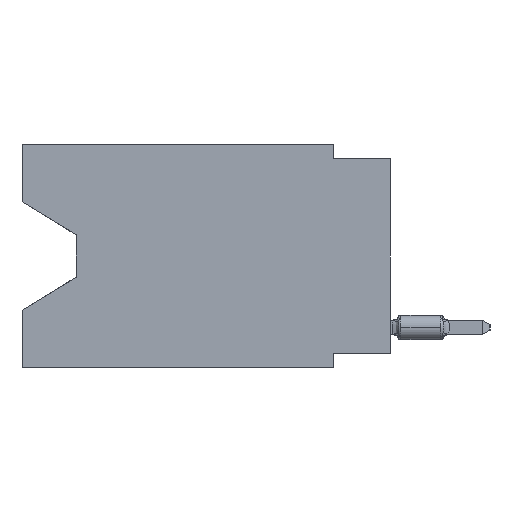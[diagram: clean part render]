
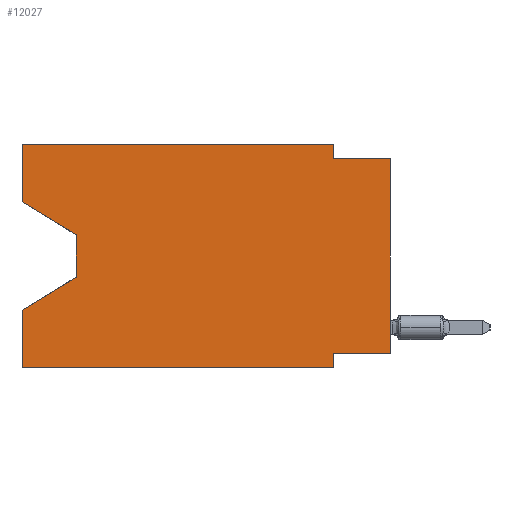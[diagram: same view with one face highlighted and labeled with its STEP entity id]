
A CAD part, left-side view. The second image highlights one B-rep face of the part: STEP entity #12027.
In plain terms, the highlighted planar face has unit normal (-1, 0, 0).
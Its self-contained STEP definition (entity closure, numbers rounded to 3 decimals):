
#24 = EDGE_CURVE ( 'NONE', #1278, #14343, #8043, .T. ) ;
#43 = CARTESIAN_POINT ( 'NONE',  ( 0., 13.97, -4.013 ) ) ;
#443 = ORIENTED_EDGE ( 'NONE', *, *, #35707, .T. ) ;
#449 = CARTESIAN_POINT ( 'NONE',  ( 0., 16.383, 0. ) ) ;
#1278 = VERTEX_POINT ( 'NONE', #25977 ) ;
#2198 = EDGE_CURVE ( 'NONE', #7456, #37600, #7278, .T. ) ;
#2207 = CARTESIAN_POINT ( 'NONE',  ( 0., 0., -0.635 ) ) ;
#2524 = EDGE_CURVE ( 'NONE', #11886, #22680, #27853, .T. ) ;
#3757 = LINE ( 'NONE', #13582, #19333 ) ;
#3829 = CARTESIAN_POINT ( 'NONE',  ( 0., 16.383, 0. ) ) ;
#4867 = LINE ( 'NONE', #16877, #7939 ) ;
#5204 = EDGE_CURVE ( 'NONE', #37988, #37600, #23819, .T. ) ;
#5759 = VECTOR ( 'NONE', #25154, 1000. ) ;
#5802 = ORIENTED_EDGE ( 'NONE', *, *, #24, .F. ) ;
#7278 = LINE ( 'NONE', #22023, #5759 ) ;
#7456 = VERTEX_POINT ( 'NONE', #24788 ) ;
#7939 = VECTOR ( 'NONE', #10017, 1000. ) ;
#8043 = LINE ( 'NONE', #32368, #18866 ) ;
#8679 = VERTEX_POINT ( 'NONE', #33979 ) ;
#8812 = LINE ( 'NONE', #21389, #20976 ) ;
#9081 = LINE ( 'NONE', #29108, #38575 ) ;
#9101 = LINE ( 'NONE', #24217, #18925 ) ;
#9214 = DIRECTION ( 'NONE',  ( 0., 0., -1. ) ) ;
#10017 = DIRECTION ( 'NONE',  ( 0., -0.855, -0.519 ) ) ;
#11312 = EDGE_CURVE ( 'NONE', #11886, #8679, #4867, .T. ) ;
#11886 = VERTEX_POINT ( 'NONE', #22898 ) ;
#12027 = ADVANCED_FACE ( 'NONE', ( #29937 ), #12666, .F. ) ;
#12666 = PLANE ( 'NONE',  #12703 ) ;
#12680 = CARTESIAN_POINT ( 'NONE',  ( 0., 2.54, -9.271 ) ) ;
#12703 = AXIS2_PLACEMENT_3D ( 'NONE', #449, #24246, #30527 ) ;
#13582 = CARTESIAN_POINT ( 'NONE',  ( 0., 0., -9.271 ) ) ;
#14343 = VERTEX_POINT ( 'NONE', #19339 ) ;
#14883 = VECTOR ( 'NONE', #36579, 1000. ) ;
#15309 = DIRECTION ( 'NONE',  ( 0., 0., 1. ) ) ;
#15353 = EDGE_LOOP ( 'NONE', ( #17076, #443, #38571, #5802, #32277, #36869, #23193, #25062, #33056, #28447, #30526, #15473 ) ) ;
#15473 = ORIENTED_EDGE ( 'NONE', *, *, #2524, .F. ) ;
#15837 = DIRECTION ( 'NONE',  ( 0., -1., 0. ) ) ;
#16877 = CARTESIAN_POINT ( 'NONE',  ( 0., 16.383, -2.546 ) ) ;
#17076 = ORIENTED_EDGE ( 'NONE', *, *, #11312, .T. ) ;
#18195 = VERTEX_POINT ( 'NONE', #12680 ) ;
#18658 = CARTESIAN_POINT ( 'NONE',  ( 0., 16.383, 0. ) ) ;
#18866 = VECTOR ( 'NONE', #20043, 1000. ) ;
#18925 = VECTOR ( 'NONE', #33028, 1000. ) ;
#19333 = VECTOR ( 'NONE', #31246, 1000. ) ;
#19339 = CARTESIAN_POINT ( 'NONE',  ( 0., 16.383, -7.36 ) ) ;
#19644 = VECTOR ( 'NONE', #15837, 1000. ) ;
#19868 = CARTESIAN_POINT ( 'NONE',  ( 0., 2.54, -0.635 ) ) ;
#20043 = DIRECTION ( 'NONE',  ( 0., 0., 1. ) ) ;
#20976 = VECTOR ( 'NONE', #9214, 1000. ) ;
#21363 = CARTESIAN_POINT ( 'NONE',  ( 0., 13.97, -5.893 ) ) ;
#21389 = CARTESIAN_POINT ( 'NONE',  ( 0., 2.54, 0. ) ) ;
#22023 = CARTESIAN_POINT ( 'NONE',  ( 0., 0., 0. ) ) ;
#22624 = EDGE_CURVE ( 'NONE', #22680, #35883, #31307, .T. ) ;
#22680 = VERTEX_POINT ( 'NONE', #31878 ) ;
#22898 = CARTESIAN_POINT ( 'NONE',  ( 0., 16.383, -2.546 ) ) ;
#23029 = CARTESIAN_POINT ( 'NONE',  ( 0., 2.54, 0. ) ) ;
#23193 = ORIENTED_EDGE ( 'NONE', *, *, #37741, .F. ) ;
#23819 = LINE ( 'NONE', #2207, #29844 ) ;
#24037 = DIRECTION ( 'NONE',  ( 0., 0., -1. ) ) ;
#24217 = CARTESIAN_POINT ( 'NONE',  ( 0., 13.97, -5.893 ) ) ;
#24246 = DIRECTION ( 'NONE',  ( 1., 0., 0. ) ) ;
#24788 = CARTESIAN_POINT ( 'NONE',  ( 0., 0., -9.271 ) ) ;
#25038 = LINE ( 'NONE', #36778, #14883 ) ;
#25062 = ORIENTED_EDGE ( 'NONE', *, *, #2198, .T. ) ;
#25154 = DIRECTION ( 'NONE',  ( 0., 0., 1. ) ) ;
#25977 = CARTESIAN_POINT ( 'NONE',  ( 0., 16.383, -9.906 ) ) ;
#26968 = LINE ( 'NONE', #43, #29199 ) ;
#27542 = EDGE_CURVE ( 'NONE', #18195, #31358, #9081, .T. ) ;
#27853 = LINE ( 'NONE', #18658, #37751 ) ;
#28447 = ORIENTED_EDGE ( 'NONE', *, *, #33686, .F. ) ;
#28996 = VERTEX_POINT ( 'NONE', #21363 ) ;
#29108 = CARTESIAN_POINT ( 'NONE',  ( 0., 2.54, -9.906 ) ) ;
#29120 = DIRECTION ( 'NONE',  ( 0., -1., 0. ) ) ;
#29199 = VECTOR ( 'NONE', #24037, 1000. ) ;
#29477 = DIRECTION ( 'NONE',  ( 0., 0., -1. ) ) ;
#29500 = EDGE_CURVE ( 'NONE', #1278, #31358, #25038, .T. ) ;
#29844 = VECTOR ( 'NONE', #29120, 1000. ) ;
#29937 = FACE_OUTER_BOUND ( 'NONE', #15353, .T. ) ;
#30046 = CARTESIAN_POINT ( 'NONE',  ( 0., 2.54, -9.906 ) ) ;
#30526 = ORIENTED_EDGE ( 'NONE', *, *, #22624, .F. ) ;
#30527 = DIRECTION ( 'NONE',  ( 0., 0., -1. ) ) ;
#31246 = DIRECTION ( 'NONE',  ( 0., 1., 0. ) ) ;
#31307 = LINE ( 'NONE', #3829, #19644 ) ;
#31358 = VERTEX_POINT ( 'NONE', #30046 ) ;
#31878 = CARTESIAN_POINT ( 'NONE',  ( 0., 16.383, 0. ) ) ;
#32277 = ORIENTED_EDGE ( 'NONE', *, *, #29500, .T. ) ;
#32368 = CARTESIAN_POINT ( 'NONE',  ( 0., 16.383, 0. ) ) ;
#32826 = EDGE_CURVE ( 'NONE', #28996, #14343, #9101, .T. ) ;
#33028 = DIRECTION ( 'NONE',  ( 0., 0.855, -0.519 ) ) ;
#33056 = ORIENTED_EDGE ( 'NONE', *, *, #5204, .F. ) ;
#33686 = EDGE_CURVE ( 'NONE', #35883, #37988, #8812, .T. ) ;
#33979 = CARTESIAN_POINT ( 'NONE',  ( 0., 13.97, -4.013 ) ) ;
#34962 = CARTESIAN_POINT ( 'NONE',  ( 0., 0., -0.635 ) ) ;
#35707 = EDGE_CURVE ( 'NONE', #8679, #28996, #26968, .T. ) ;
#35883 = VERTEX_POINT ( 'NONE', #23029 ) ;
#36579 = DIRECTION ( 'NONE',  ( 0., -1., 0. ) ) ;
#36778 = CARTESIAN_POINT ( 'NONE',  ( 0., 16.383, -9.906 ) ) ;
#36869 = ORIENTED_EDGE ( 'NONE', *, *, #27542, .F. ) ;
#37600 = VERTEX_POINT ( 'NONE', #34962 ) ;
#37741 = EDGE_CURVE ( 'NONE', #7456, #18195, #3757, .T. ) ;
#37751 = VECTOR ( 'NONE', #15309, 1000. ) ;
#37988 = VERTEX_POINT ( 'NONE', #19868 ) ;
#38571 = ORIENTED_EDGE ( 'NONE', *, *, #32826, .T. ) ;
#38575 = VECTOR ( 'NONE', #29477, 1000. ) ;
